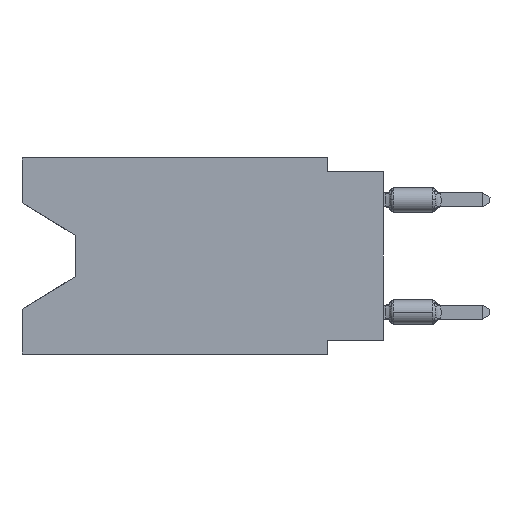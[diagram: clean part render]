
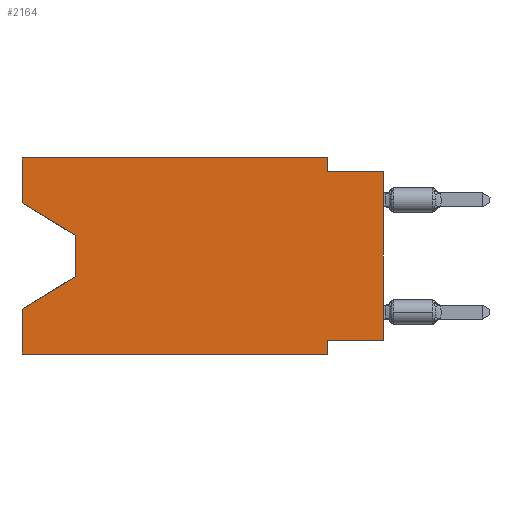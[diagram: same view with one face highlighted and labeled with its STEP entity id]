
A CAD part, left-side view. The second image highlights one B-rep face of the part: STEP entity #2164.
In plain terms, the highlighted planar face has unit normal (-1, 0, 0).
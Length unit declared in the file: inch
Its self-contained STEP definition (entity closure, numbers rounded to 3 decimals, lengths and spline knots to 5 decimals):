
#51 = CARTESIAN_POINT ( 'NONE',  ( 0., 0.1, -0.025 ) ) ;
#183 = VERTEX_POINT ( 'NONE', #11848 ) ;
#211 = LINE ( 'NONE', #8176, #15887 ) ;
#283 = ORIENTED_EDGE ( 'NONE', *, *, #9556, .T. ) ;
#301 = DIRECTION ( 'NONE',  ( 1., 0., 0. ) ) ;
#415 = DIRECTION ( 'NONE',  ( 0., 0., -1. ) ) ;
#457 = CARTESIAN_POINT ( 'NONE',  ( 0., 0.1, -0.35 ) ) ;
#1105 = CARTESIAN_POINT ( 'NONE',  ( 0., 0.645, -0.35 ) ) ;
#1273 = EDGE_CURVE ( 'NONE', #183, #10645, #14300, .T. ) ;
#1575 = EDGE_CURVE ( 'NONE', #12644, #15400, #7967, .T. ) ;
#1599 = EDGE_CURVE ( 'NONE', #15324, #11745, #8572, .T. ) ;
#1953 = ORIENTED_EDGE ( 'NONE', *, *, #13597, .F. ) ;
#2099 = VECTOR ( 'NONE', #17791, 39.37008 ) ;
#2118 = CARTESIAN_POINT ( 'NONE',  ( 0., 0.55, -0.212 ) ) ;
#2164 = ADVANCED_FACE ( 'NONE', ( #15357 ), #15453, .F. ) ;
#3129 = CARTESIAN_POINT ( 'NONE',  ( 0., 0.645, 0. ) ) ;
#3367 = CARTESIAN_POINT ( 'NONE',  ( 0., 0.1, -0.35 ) ) ;
#3833 = LINE ( 'NONE', #6756, #9548 ) ;
#3968 = AXIS2_PLACEMENT_3D ( 'NONE', #3129, #301, #12520 ) ;
#4024 = CARTESIAN_POINT ( 'NONE',  ( 0., 0.645, -0.08025 ) ) ;
#4687 = EDGE_CURVE ( 'NONE', #12644, #12779, #7550, .T. ) ;
#5150 = CARTESIAN_POINT ( 'NONE',  ( 0., 0., -0.325 ) ) ;
#5227 = CARTESIAN_POINT ( 'NONE',  ( 0., 0.645, 0. ) ) ;
#5297 = EDGE_CURVE ( 'NONE', #9853, #11745, #16203, .T. ) ;
#5344 = LINE ( 'NONE', #11409, #9691 ) ;
#5478 = DIRECTION ( 'NONE',  ( 0., 0., 1. ) ) ;
#5534 = EDGE_CURVE ( 'NONE', #15400, #6791, #12451, .T. ) ;
#5598 = LINE ( 'NONE', #5150, #13783 ) ;
#5640 = VECTOR ( 'NONE', #14043, 39.37008 ) ;
#6321 = ORIENTED_EDGE ( 'NONE', *, *, #7080, .T. ) ;
#6756 = CARTESIAN_POINT ( 'NONE',  ( 0., 0.1, 0. ) ) ;
#6791 = VERTEX_POINT ( 'NONE', #12236 ) ;
#7080 = EDGE_CURVE ( 'NONE', #9853, #10645, #14748, .T. ) ;
#7550 = LINE ( 'NONE', #16957, #13493 ) ;
#7614 = EDGE_CURVE ( 'NONE', #12847, #19436, #18628, .T. ) ;
#7659 = VERTEX_POINT ( 'NONE', #51 ) ;
#7727 = ORIENTED_EDGE ( 'NONE', *, *, #1599, .T. ) ;
#7755 = ORIENTED_EDGE ( 'NONE', *, *, #18005, .F. ) ;
#7868 = CARTESIAN_POINT ( 'NONE',  ( 0., 0.645, 0. ) ) ;
#7967 = LINE ( 'NONE', #7868, #5640 ) ;
#8176 = CARTESIAN_POINT ( 'NONE',  ( 0., 0.55, -0.138 ) ) ;
#8572 = LINE ( 'NONE', #2118, #17592 ) ;
#9548 = VECTOR ( 'NONE', #415, 39.37008 ) ;
#9556 = EDGE_CURVE ( 'NONE', #12779, #15324, #211, .T. ) ;
#9573 = CARTESIAN_POINT ( 'NONE',  ( 0., 0.55, -0.212 ) ) ;
#9691 = VECTOR ( 'NONE', #19092, 39.37008 ) ;
#9712 = DIRECTION ( 'NONE',  ( 0., -1., 0. ) ) ;
#9801 = CARTESIAN_POINT ( 'NONE',  ( 0., 0.645, -0.35 ) ) ;
#9853 = VERTEX_POINT ( 'NONE', #1105 ) ;
#10556 = CARTESIAN_POINT ( 'NONE',  ( 0., 0.645, -0.26975 ) ) ;
#10645 = VERTEX_POINT ( 'NONE', #3367 ) ;
#11043 = ORIENTED_EDGE ( 'NONE', *, *, #1273, .F. ) ;
#11201 = DIRECTION ( 'NONE',  ( 0., 0.855, -0.519 ) ) ;
#11409 = CARTESIAN_POINT ( 'NONE',  ( 0., 0., -0.025 ) ) ;
#11454 = CARTESIAN_POINT ( 'NONE',  ( 0., 0.645, 0. ) ) ;
#11745 = VERTEX_POINT ( 'NONE', #10556 ) ;
#11848 = CARTESIAN_POINT ( 'NONE',  ( 0., 0.1, -0.325 ) ) ;
#12236 = CARTESIAN_POINT ( 'NONE',  ( 0., 0.1, 0. ) ) ;
#12278 = ORIENTED_EDGE ( 'NONE', *, *, #4687, .T. ) ;
#12371 = CARTESIAN_POINT ( 'NONE',  ( 0., 0., 0. ) ) ;
#12387 = EDGE_LOOP ( 'NONE', ( #12278, #283, #7727, #19883, #6321, #11043, #13435, #14608, #1953, #7755, #14858, #18847 ) ) ;
#12451 = LINE ( 'NONE', #17392, #18223 ) ;
#12520 = DIRECTION ( 'NONE',  ( 0., 0., -1. ) ) ;
#12644 = VERTEX_POINT ( 'NONE', #4024 ) ;
#12740 = DIRECTION ( 'NONE',  ( 0., 1., 0. ) ) ;
#12779 = VERTEX_POINT ( 'NONE', #18270 ) ;
#12847 = VERTEX_POINT ( 'NONE', #14215 ) ;
#13435 = ORIENTED_EDGE ( 'NONE', *, *, #17617, .F. ) ;
#13493 = VECTOR ( 'NONE', #16854, 39.37008 ) ;
#13597 = EDGE_CURVE ( 'NONE', #7659, #19436, #5344, .T. ) ;
#13783 = VECTOR ( 'NONE', #12740, 39.37008 ) ;
#14028 = CARTESIAN_POINT ( 'NONE',  ( 0., 0., -0.025 ) ) ;
#14043 = DIRECTION ( 'NONE',  ( 0., 0., 1. ) ) ;
#14215 = CARTESIAN_POINT ( 'NONE',  ( 0., 0., -0.325 ) ) ;
#14300 = LINE ( 'NONE', #457, #2099 ) ;
#14545 = DIRECTION ( 'NONE',  ( 0., -1., 0. ) ) ;
#14608 = ORIENTED_EDGE ( 'NONE', *, *, #7614, .T. ) ;
#14748 = LINE ( 'NONE', #9801, #19757 ) ;
#14858 = ORIENTED_EDGE ( 'NONE', *, *, #5534, .F. ) ;
#15324 = VERTEX_POINT ( 'NONE', #9573 ) ;
#15357 = FACE_OUTER_BOUND ( 'NONE', #12387, .T. ) ;
#15400 = VERTEX_POINT ( 'NONE', #5227 ) ;
#15453 = PLANE ( 'NONE',  #3968 ) ;
#15887 = VECTOR ( 'NONE', #18580, 39.37008 ) ;
#15897 = VECTOR ( 'NONE', #18531, 39.37008 ) ;
#15973 = VECTOR ( 'NONE', #5478, 39.37008 ) ;
#16203 = LINE ( 'NONE', #11454, #15973 ) ;
#16854 = DIRECTION ( 'NONE',  ( 0., -0.855, -0.519 ) ) ;
#16957 = CARTESIAN_POINT ( 'NONE',  ( 0., 0.645, -0.08025 ) ) ;
#17392 = CARTESIAN_POINT ( 'NONE',  ( 0., 0.645, 0. ) ) ;
#17592 = VECTOR ( 'NONE', #11201, 39.37008 ) ;
#17617 = EDGE_CURVE ( 'NONE', #12847, #183, #5598, .T. ) ;
#17791 = DIRECTION ( 'NONE',  ( 0., 0., -1. ) ) ;
#18005 = EDGE_CURVE ( 'NONE', #6791, #7659, #3833, .T. ) ;
#18223 = VECTOR ( 'NONE', #9712, 39.37008 ) ;
#18270 = CARTESIAN_POINT ( 'NONE',  ( 0., 0.55, -0.138 ) ) ;
#18531 = DIRECTION ( 'NONE',  ( 0., 0., 1. ) ) ;
#18580 = DIRECTION ( 'NONE',  ( 0., 0., -1. ) ) ;
#18628 = LINE ( 'NONE', #12371, #15897 ) ;
#18847 = ORIENTED_EDGE ( 'NONE', *, *, #1575, .F. ) ;
#19092 = DIRECTION ( 'NONE',  ( 0., -1., 0. ) ) ;
#19436 = VERTEX_POINT ( 'NONE', #14028 ) ;
#19757 = VECTOR ( 'NONE', #14545, 39.37008 ) ;
#19883 = ORIENTED_EDGE ( 'NONE', *, *, #5297, .F. ) ;
